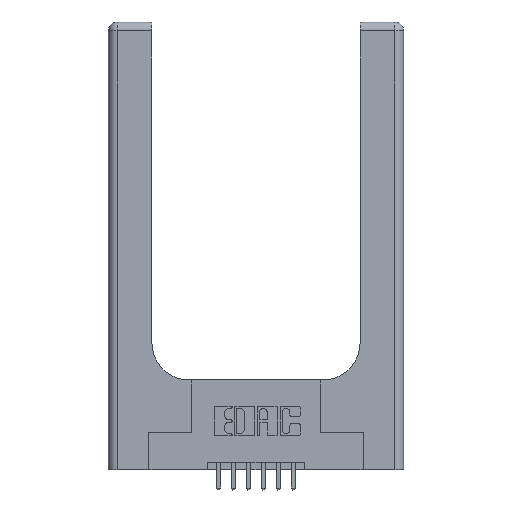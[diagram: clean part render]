
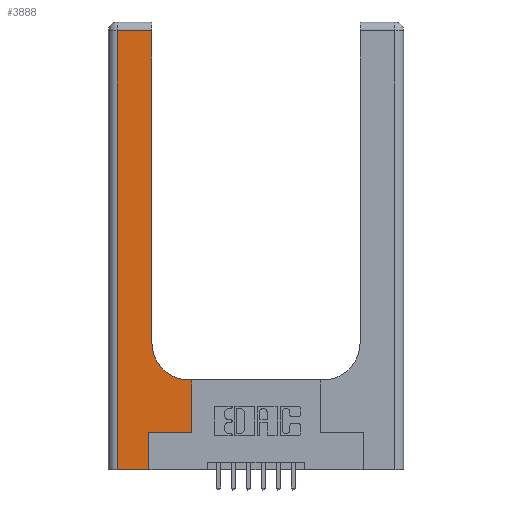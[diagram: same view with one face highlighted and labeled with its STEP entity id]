
A CAD part, top view. The second image highlights one B-rep face of the part: STEP entity #3888.
In plain terms, the highlighted planar face has unit normal (0, 0, 1).
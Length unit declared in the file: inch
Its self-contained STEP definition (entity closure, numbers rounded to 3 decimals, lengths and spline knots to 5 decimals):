
#149 = VERTEX_POINT ( 'NONE', #11397 ) ;
#178 = VECTOR ( 'NONE', #10978, 39.37008 ) ;
#525 = EDGE_CURVE ( 'NONE', #4836, #149, #7063, .T. ) ;
#626 = EDGE_CURVE ( 'NONE', #3470, #2417, #4222, .T. ) ;
#649 = ORIENTED_EDGE ( 'NONE', *, *, #9102, .T. ) ;
#666 = EDGE_CURVE ( 'NONE', #6658, #6824, #7947, .T. ) ;
#1032 = EDGE_CURVE ( 'NONE', #6824, #3451, #3866, .T. ) ;
#1072 = PLANE ( 'NONE',  #1963 ) ;
#1151 = AXIS2_PLACEMENT_3D ( 'NONE', #13451, #13348, #4334 ) ;
#1410 = CIRCLE ( 'NONE', #1151, 0.25 ) ;
#1660 = ORIENTED_EDGE ( 'NONE', *, *, #666, .T. ) ;
#1776 = DIRECTION ( 'NONE',  ( 0., 1., 0. ) ) ;
#1919 = VECTOR ( 'NONE', #1776, 39.37008 ) ;
#1963 = AXIS2_PLACEMENT_3D ( 'NONE', #14504, #2125, #12354 ) ;
#1983 = ORIENTED_EDGE ( 'NONE', *, *, #525, .T. ) ;
#2125 = DIRECTION ( 'NONE',  ( 0., 0., -1. ) ) ;
#2172 = EDGE_CURVE ( 'NONE', #3451, #7834, #12891, .T. ) ;
#2273 = VERTEX_POINT ( 'NONE', #3553 ) ;
#2417 = VERTEX_POINT ( 'NONE', #3746 ) ;
#2710 = CARTESIAN_POINT ( 'NONE',  ( 0.5585, 0.25, 0.37 ) ) ;
#2813 = DIRECTION ( 'NONE',  ( -1., 0., 0. ) ) ;
#2879 = FACE_OUTER_BOUND ( 'NONE', #12840, .T. ) ;
#3411 = CARTESIAN_POINT ( 'NONE',  ( 0.06, 3., 0.37 ) ) ;
#3451 = VERTEX_POINT ( 'NONE', #9131 ) ;
#3470 = VERTEX_POINT ( 'NONE', #4893 ) ;
#3553 = CARTESIAN_POINT ( 'NONE',  ( 0.269, 0., 0.37 ) ) ;
#3629 = EDGE_CURVE ( 'NONE', #2417, #4836, #10546, .T. ) ;
#3746 = CARTESIAN_POINT ( 'NONE',  ( 0.5585, 0.25, 0.37 ) ) ;
#3837 = LINE ( 'NONE', #8525, #12188 ) ;
#3866 = LINE ( 'NONE', #14214, #14553 ) ;
#3888 = ADVANCED_FACE ( 'NONE', ( #2879 ), #1072, .F. ) ;
#3952 = DIRECTION ( 'NONE',  ( 0., 1., 0. ) ) ;
#4028 = CARTESIAN_POINT ( 'NONE',  ( 0.2915, 2.94, 0.37 ) ) ;
#4036 = VECTOR ( 'NONE', #12529, 39.37008 ) ;
#4164 = ORIENTED_EDGE ( 'NONE', *, *, #3629, .T. ) ;
#4222 = LINE ( 'NONE', #6138, #7256 ) ;
#4281 = LINE ( 'NONE', #9795, #178 ) ;
#4334 = DIRECTION ( 'NONE',  ( 1., 0., 0. ) ) ;
#4484 = CARTESIAN_POINT ( 'NONE',  ( 0.5585, 0.6, 0.37 ) ) ;
#4697 = ORIENTED_EDGE ( 'NONE', *, *, #7949, .T. ) ;
#4836 = VERTEX_POINT ( 'NONE', #4484 ) ;
#4893 = CARTESIAN_POINT ( 'NONE',  ( 0.269, 0.25, 0.37 ) ) ;
#5102 = CARTESIAN_POINT ( 'NONE',  ( 0.06, 0., 0.37 ) ) ;
#6138 = CARTESIAN_POINT ( 'NONE',  ( 0.269, 0.25, 0.37 ) ) ;
#6658 = VERTEX_POINT ( 'NONE', #6876 ) ;
#6824 = VERTEX_POINT ( 'NONE', #4028 ) ;
#6876 = CARTESIAN_POINT ( 'NONE',  ( 0.2915, 0.85, 0.37 ) ) ;
#7063 = LINE ( 'NONE', #10240, #4036 ) ;
#7256 = VECTOR ( 'NONE', #11948, 39.37008 ) ;
#7834 = VERTEX_POINT ( 'NONE', #5102 ) ;
#7947 = LINE ( 'NONE', #8417, #1919 ) ;
#7949 = EDGE_CURVE ( 'NONE', #7834, #2273, #4281, .T. ) ;
#7987 = DIRECTION ( 'NONE',  ( 0., -1., 0. ) ) ;
#8079 = ORIENTED_EDGE ( 'NONE', *, *, #626, .T. ) ;
#8417 = CARTESIAN_POINT ( 'NONE',  ( 0.2915, 3., 0.37 ) ) ;
#8525 = CARTESIAN_POINT ( 'NONE',  ( 0.269, 0., 0.37 ) ) ;
#8569 = VECTOR ( 'NONE', #3952, 39.37008 ) ;
#8593 = ORIENTED_EDGE ( 'NONE', *, *, #2172, .T. ) ;
#9102 = EDGE_CURVE ( 'NONE', #149, #6658, #1410, .T. ) ;
#9131 = CARTESIAN_POINT ( 'NONE',  ( 0.06, 2.94, 0.37 ) ) ;
#9795 = CARTESIAN_POINT ( 'NONE',  ( 0., 0., 0.37 ) ) ;
#9879 = ORIENTED_EDGE ( 'NONE', *, *, #12113, .T. ) ;
#10240 = CARTESIAN_POINT ( 'NONE',  ( 0.2915, 0.6, 0.37 ) ) ;
#10546 = LINE ( 'NONE', #2710, #8569 ) ;
#10820 = DIRECTION ( 'NONE',  ( 0., 1., 0. ) ) ;
#10978 = DIRECTION ( 'NONE',  ( 1., 0., 0. ) ) ;
#11397 = CARTESIAN_POINT ( 'NONE',  ( 0.5415, 0.6, 0.37 ) ) ;
#11948 = DIRECTION ( 'NONE',  ( 1., 0., 0. ) ) ;
#12113 = EDGE_CURVE ( 'NONE', #2273, #3470, #3837, .T. ) ;
#12188 = VECTOR ( 'NONE', #10820, 39.37008 ) ;
#12354 = DIRECTION ( 'NONE',  ( -1., 0., 0. ) ) ;
#12529 = DIRECTION ( 'NONE',  ( -1., 0., 0. ) ) ;
#12840 = EDGE_LOOP ( 'NONE', ( #1660, #14319, #8593, #4697, #9879, #8079, #4164, #1983, #649 ) ) ;
#12891 = LINE ( 'NONE', #3411, #13972 ) ;
#13348 = DIRECTION ( 'NONE',  ( 0., 0., -1. ) ) ;
#13451 = CARTESIAN_POINT ( 'NONE',  ( 0.5415, 0.85, 0.37 ) ) ;
#13972 = VECTOR ( 'NONE', #7987, 39.37008 ) ;
#14214 = CARTESIAN_POINT ( 'NONE',  ( 0., 2.94, 0.37 ) ) ;
#14319 = ORIENTED_EDGE ( 'NONE', *, *, #1032, .T. ) ;
#14504 = CARTESIAN_POINT ( 'NONE',  ( 0., 3., 0.37 ) ) ;
#14553 = VECTOR ( 'NONE', #2813, 39.37008 ) ;
